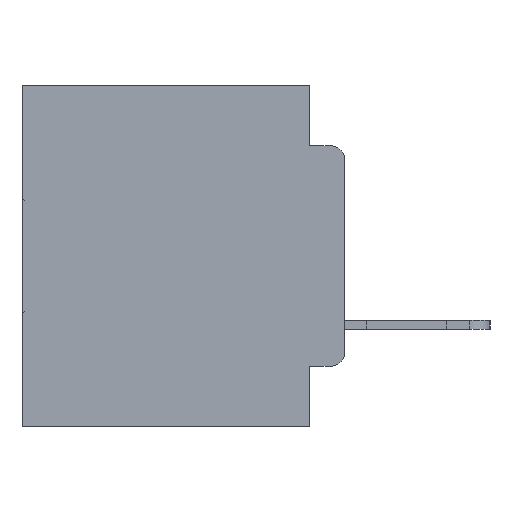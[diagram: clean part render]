
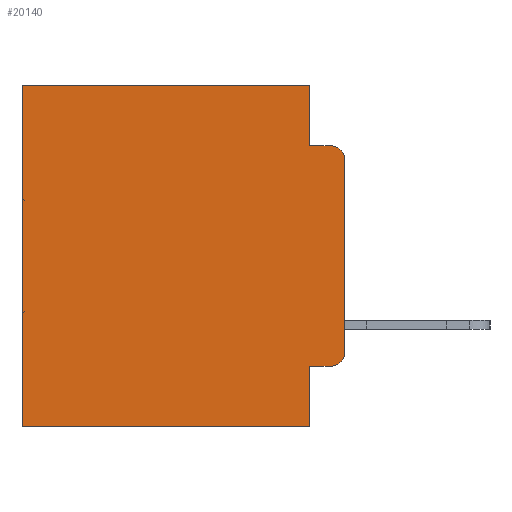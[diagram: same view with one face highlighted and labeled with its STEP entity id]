
A CAD part, left-side view. The second image highlights one B-rep face of the part: STEP entity #20140.
In plain terms, the highlighted planar face has unit normal (-1, 0, 0).
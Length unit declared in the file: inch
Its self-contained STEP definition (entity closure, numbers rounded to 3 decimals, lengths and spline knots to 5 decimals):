
#321 = DIRECTION ( 'NONE',  ( 0., 0., -1. ) ) ;
#528 = CARTESIAN_POINT ( 'NONE',  ( 0.298, 0.051, -0.4115 ) ) ;
#588 = DIRECTION ( 'NONE',  ( 0., 0., -1. ) ) ;
#2008 = ORIENTED_EDGE ( 'NONE', *, *, #23654, .F. ) ;
#2049 = AXIS2_PLACEMENT_3D ( 'NONE', #28001, #15782, #588 ) ;
#2387 = LINE ( 'NONE', #31741, #28107 ) ;
#2718 = ORIENTED_EDGE ( 'NONE', *, *, #11064, .T. ) ;
#3385 = VECTOR ( 'NONE', #15553, 39.37008 ) ;
#3453 = ORIENTED_EDGE ( 'NONE', *, *, #13858, .T. ) ;
#3695 = DIRECTION ( 'NONE',  ( 0., 0., -1. ) ) ;
#4282 = LINE ( 'NONE', #12980, #9391 ) ;
#4401 = CARTESIAN_POINT ( 'NONE',  ( 0.298, 0.02, -0.1085 ) ) ;
#4653 = ORIENTED_EDGE ( 'NONE', *, *, #27148, .F. ) ;
#5246 = VECTOR ( 'NONE', #21337, 39.37008 ) ;
#5690 = AXIS2_PLACEMENT_3D ( 'NONE', #30730, #30504, #30637 ) ;
#7205 = VECTOR ( 'NONE', #11889, 39.37008 ) ;
#7368 = VERTEX_POINT ( 'NONE', #21382 ) ;
#7409 = CARTESIAN_POINT ( 'NONE',  ( 0.298, 0., -0.5 ) ) ;
#9179 = AXIS2_PLACEMENT_3D ( 'NONE', #4401, #27858, #3695 ) ;
#9391 = VECTOR ( 'NONE', #15582, 39.37008 ) ;
#9749 = LINE ( 'NONE', #31523, #16558 ) ;
#10621 = PLANE ( 'NONE',  #2049 ) ;
#10765 = CARTESIAN_POINT ( 'NONE',  ( 0.298, 0.02, -0.4115 ) ) ;
#11064 = EDGE_CURVE ( 'NONE', #14287, #24039, #13935, .T. ) ;
#11563 = VECTOR ( 'NONE', #15733, 39.37008 ) ;
#11606 = EDGE_CURVE ( 'NONE', #12627, #19713, #26002, .T. ) ;
#11809 = CIRCLE ( 'NONE', #5690, 0.02 ) ;
#11889 = DIRECTION ( 'NONE',  ( 0., 1., 0. ) ) ;
#12627 = VERTEX_POINT ( 'NONE', #20053 ) ;
#12704 = VERTEX_POINT ( 'NONE', #30963 ) ;
#12980 = CARTESIAN_POINT ( 'NONE',  ( 0.298, 0.051, 0. ) ) ;
#13636 = CARTESIAN_POINT ( 'NONE',  ( 0.298, 0.02, -0.0885 ) ) ;
#13744 = EDGE_CURVE ( 'NONE', #22301, #19713, #2387, .T. ) ;
#13858 = EDGE_CURVE ( 'NONE', #15538, #12704, #11809, .T. ) ;
#13935 = LINE ( 'NONE', #26558, #7205 ) ;
#14287 = VERTEX_POINT ( 'NONE', #19435 ) ;
#14589 = ORIENTED_EDGE ( 'NONE', *, *, #23847, .T. ) ;
#14704 = EDGE_LOOP ( 'NONE', ( #25182, #15391, #28012, #4653, #2718, #22453, #20238, #2008, #14589, #3453 ) ) ;
#14974 = EDGE_CURVE ( 'NONE', #12627, #12704, #9749, .T. ) ;
#15135 = CARTESIAN_POINT ( 'NONE',  ( 0.298, 0.473, -0.5 ) ) ;
#15391 = ORIENTED_EDGE ( 'NONE', *, *, #11606, .T. ) ;
#15538 = VERTEX_POINT ( 'NONE', #10765 ) ;
#15553 = DIRECTION ( 'NONE',  ( 0., 0., -1. ) ) ;
#15582 = DIRECTION ( 'NONE',  ( 0., 0., -1. ) ) ;
#15733 = DIRECTION ( 'NONE',  ( 0., 0., -1. ) ) ;
#15782 = DIRECTION ( 'NONE',  ( 1., 0., 0. ) ) ;
#16412 = LINE ( 'NONE', #7409, #21496 ) ;
#16558 = VECTOR ( 'NONE', #321, 39.37008 ) ;
#16882 = FACE_OUTER_BOUND ( 'NONE', #14704, .T. ) ;
#19435 = CARTESIAN_POINT ( 'NONE',  ( 0.298, 0.051, 0. ) ) ;
#19713 = VERTEX_POINT ( 'NONE', #13636 ) ;
#20053 = CARTESIAN_POINT ( 'NONE',  ( 0.298, 0., -0.1085 ) ) ;
#20140 = ADVANCED_FACE ( 'NONE', ( #16882 ), #10621, .F. ) ;
#20238 = ORIENTED_EDGE ( 'NONE', *, *, #23495, .F. ) ;
#21337 = DIRECTION ( 'NONE',  ( 0., -1., 0. ) ) ;
#21382 = CARTESIAN_POINT ( 'NONE',  ( 0.298, 0.051, -0.5 ) ) ;
#21496 = VECTOR ( 'NONE', #27358, 39.37008 ) ;
#22091 = CARTESIAN_POINT ( 'NONE',  ( 0.298, 0.473, 0. ) ) ;
#22301 = VERTEX_POINT ( 'NONE', #27318 ) ;
#22453 = ORIENTED_EDGE ( 'NONE', *, *, #29707, .T. ) ;
#23403 = LINE ( 'NONE', #28583, #5246 ) ;
#23495 = EDGE_CURVE ( 'NONE', #7368, #24171, #16412, .T. ) ;
#23654 = EDGE_CURVE ( 'NONE', #32040, #7368, #29720, .T. ) ;
#23847 = EDGE_CURVE ( 'NONE', #32040, #15538, #23403, .T. ) ;
#24039 = VERTEX_POINT ( 'NONE', #22091 ) ;
#24171 = VERTEX_POINT ( 'NONE', #15135 ) ;
#25182 = ORIENTED_EDGE ( 'NONE', *, *, #14974, .F. ) ;
#26002 = CIRCLE ( 'NONE', #9179, 0.02 ) ;
#26558 = CARTESIAN_POINT ( 'NONE',  ( 0.298, 0., 0. ) ) ;
#27148 = EDGE_CURVE ( 'NONE', #14287, #22301, #4282, .T. ) ;
#27318 = CARTESIAN_POINT ( 'NONE',  ( 0.298, 0.051, -0.0885 ) ) ;
#27358 = DIRECTION ( 'NONE',  ( 0., 1., 0. ) ) ;
#27858 = DIRECTION ( 'NONE',  ( -1., 0., 0. ) ) ;
#28001 = CARTESIAN_POINT ( 'NONE',  ( 0.298, 0., 0. ) ) ;
#28012 = ORIENTED_EDGE ( 'NONE', *, *, #13744, .F. ) ;
#28107 = VECTOR ( 'NONE', #30799, 39.37008 ) ;
#28583 = CARTESIAN_POINT ( 'NONE',  ( 0.298, 0.051, -0.4115 ) ) ;
#29062 = LINE ( 'NONE', #30150, #3385 ) ;
#29707 = EDGE_CURVE ( 'NONE', #24039, #24171, #29062, .T. ) ;
#29720 = LINE ( 'NONE', #30314, #11563 ) ;
#30150 = CARTESIAN_POINT ( 'NONE',  ( 0.298, 0.473, 0. ) ) ;
#30314 = CARTESIAN_POINT ( 'NONE',  ( 0.298, 0.051, 0. ) ) ;
#30504 = DIRECTION ( 'NONE',  ( -1., 0., 0. ) ) ;
#30637 = DIRECTION ( 'NONE',  ( 0., 0., -1. ) ) ;
#30730 = CARTESIAN_POINT ( 'NONE',  ( 0.298, 0.02, -0.3915 ) ) ;
#30799 = DIRECTION ( 'NONE',  ( 0., -1., 0. ) ) ;
#30963 = CARTESIAN_POINT ( 'NONE',  ( 0.298, 0., -0.3915 ) ) ;
#31523 = CARTESIAN_POINT ( 'NONE',  ( 0.298, 0., 0. ) ) ;
#31741 = CARTESIAN_POINT ( 'NONE',  ( 0.298, 0.051, -0.0885 ) ) ;
#32040 = VERTEX_POINT ( 'NONE', #528 ) ;
